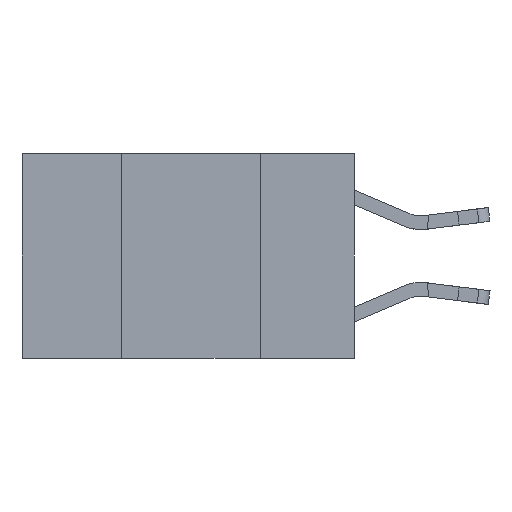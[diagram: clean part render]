
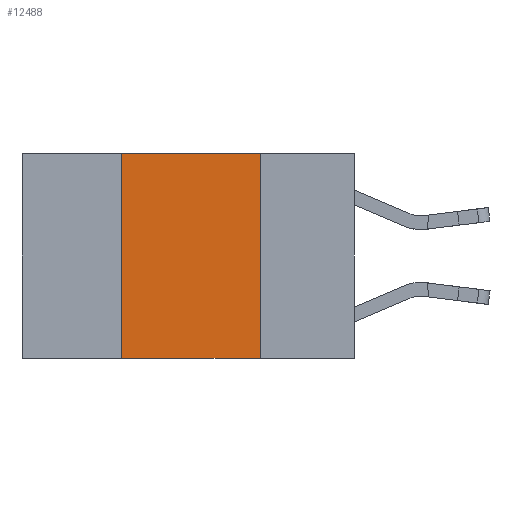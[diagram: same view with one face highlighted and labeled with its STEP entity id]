
A CAD part, left-side view. The second image highlights one B-rep face of the part: STEP entity #12488.
In plain terms, the highlighted planar face has unit normal (-1, 0, 0).
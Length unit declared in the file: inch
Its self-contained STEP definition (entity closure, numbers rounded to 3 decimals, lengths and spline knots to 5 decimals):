
#2 = CARTESIAN_POINT ( 'NONE',  ( 0., 0.17, -0.37 ) ) ;
#592 = CARTESIAN_POINT ( 'NONE',  ( 0., 0.17, 0. ) ) ;
#1868 = DIRECTION ( 'NONE',  ( 0., 0., -1. ) ) ;
#2276 = AXIS2_PLACEMENT_3D ( 'NONE', #7384, #10136, #1868 ) ;
#2357 = ORIENTED_EDGE ( 'NONE', *, *, #9956, .T. ) ;
#2472 = ORIENTED_EDGE ( 'NONE', *, *, #11086, .F. ) ;
#2635 = ORIENTED_EDGE ( 'NONE', *, *, #11723, .F. ) ;
#2793 = VERTEX_POINT ( 'NONE', #6972 ) ;
#3231 = VERTEX_POINT ( 'NONE', #592 ) ;
#3356 = VERTEX_POINT ( 'NONE', #9094 ) ;
#4244 = VECTOR ( 'NONE', #4572, 39.37008 ) ;
#4572 = DIRECTION ( 'NONE',  ( 0., 0., 1. ) ) ;
#5444 = LINE ( 'NONE', #14005, #15789 ) ;
#6972 = CARTESIAN_POINT ( 'NONE',  ( 0., 0.42, -0.37 ) ) ;
#7384 = CARTESIAN_POINT ( 'NONE',  ( 0., 0.6, 0. ) ) ;
#9094 = CARTESIAN_POINT ( 'NONE',  ( 0., 0.42, 0. ) ) ;
#9956 = EDGE_CURVE ( 'NONE', #2793, #12232, #5444, .T. ) ;
#10136 = DIRECTION ( 'NONE',  ( 1., 0., 0. ) ) ;
#10964 = DIRECTION ( 'NONE',  ( 0., -1., 0. ) ) ;
#11086 = EDGE_CURVE ( 'NONE', #3356, #3231, #16729, .T. ) ;
#11529 = LINE ( 'NONE', #16642, #4244 ) ;
#11723 = EDGE_CURVE ( 'NONE', #2793, #3356, #11529, .T. ) ;
#12232 = VERTEX_POINT ( 'NONE', #2 ) ;
#12488 = ADVANCED_FACE ( 'NONE', ( #15652 ), #15403, .F. ) ;
#12628 = EDGE_CURVE ( 'NONE', #3231, #12232, #17082, .T. ) ;
#13093 = CARTESIAN_POINT ( 'NONE',  ( 0., 0.17, 0. ) ) ;
#13621 = VECTOR ( 'NONE', #10964, 39.37008 ) ;
#13988 = EDGE_LOOP ( 'NONE', ( #17009, #2472, #2635, #2357 ) ) ;
#14005 = CARTESIAN_POINT ( 'NONE',  ( 0., 0.6, -0.37 ) ) ;
#15327 = DIRECTION ( 'NONE',  ( 0., -1., 0. ) ) ;
#15403 = PLANE ( 'NONE',  #2276 ) ;
#15652 = FACE_OUTER_BOUND ( 'NONE', #13988, .T. ) ;
#15755 = DIRECTION ( 'NONE',  ( 0., 0., -1. ) ) ;
#15789 = VECTOR ( 'NONE', #15327, 39.37008 ) ;
#16244 = VECTOR ( 'NONE', #15755, 39.37008 ) ;
#16259 = CARTESIAN_POINT ( 'NONE',  ( 0., 0.6, 0. ) ) ;
#16642 = CARTESIAN_POINT ( 'NONE',  ( 0., 0.42, 0. ) ) ;
#16729 = LINE ( 'NONE', #16259, #13621 ) ;
#17009 = ORIENTED_EDGE ( 'NONE', *, *, #12628, .F. ) ;
#17082 = LINE ( 'NONE', #13093, #16244 ) ;
